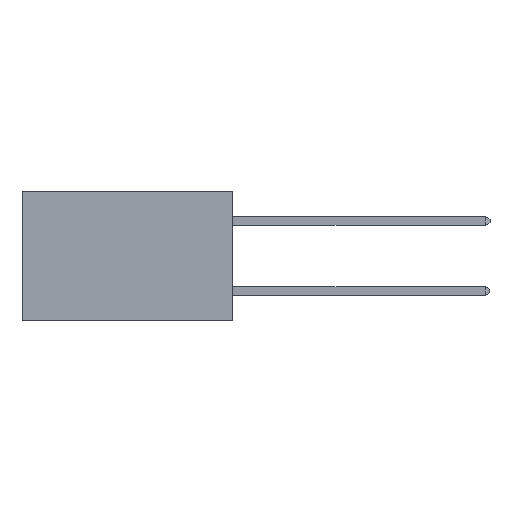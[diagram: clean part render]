
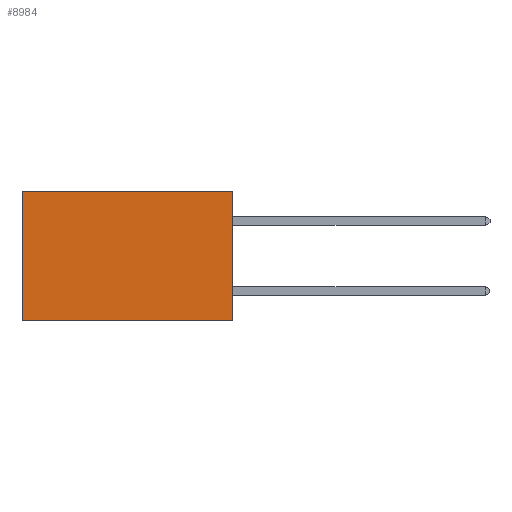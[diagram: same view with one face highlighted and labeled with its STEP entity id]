
A CAD part, left-side view. The second image highlights one B-rep face of the part: STEP entity #8984.
In plain terms, the highlighted planar face has unit normal (-1, 0, 0).
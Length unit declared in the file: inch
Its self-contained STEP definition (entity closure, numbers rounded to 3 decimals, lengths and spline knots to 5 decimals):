
#59 = FACE_OUTER_BOUND ( 'NONE', #17032, .T. ) ;
#88 = VERTEX_POINT ( 'NONE', #13013 ) ;
#177 = LINE ( 'NONE', #3454, #7431 ) ;
#2296 = DIRECTION ( 'NONE',  ( 0., 0., -1. ) ) ;
#2727 = CARTESIAN_POINT ( 'NONE',  ( 0.2875, 0.6, 0. ) ) ;
#3383 = DIRECTION ( 'NONE',  ( 0., 1., 0. ) ) ;
#3454 = CARTESIAN_POINT ( 'NONE',  ( 0.2875, 0., 0. ) ) ;
#4786 = VECTOR ( 'NONE', #8373, 39.37008 ) ;
#5776 = CARTESIAN_POINT ( 'NONE',  ( 0.2875, 0., 0. ) ) ;
#6469 = AXIS2_PLACEMENT_3D ( 'NONE', #5776, #19209, #10375 ) ;
#7085 = VERTEX_POINT ( 'NONE', #18791 ) ;
#7145 = VERTEX_POINT ( 'NONE', #17360 ) ;
#7243 = LINE ( 'NONE', #2727, #11252 ) ;
#7431 = VECTOR ( 'NONE', #3383, 39.37008 ) ;
#8373 = DIRECTION ( 'NONE',  ( 0., 1., 0. ) ) ;
#8984 = ADVANCED_FACE ( 'NONE', ( #59 ), #11770, .F. ) ;
#9493 = ORIENTED_EDGE ( 'NONE', *, *, #11775, .F. ) ;
#10375 = DIRECTION ( 'NONE',  ( 0., 0., -1. ) ) ;
#10382 = DIRECTION ( 'NONE',  ( 0., 0., -1. ) ) ;
#10971 = VECTOR ( 'NONE', #2296, 39.37008 ) ;
#11252 = VECTOR ( 'NONE', #10382, 39.37008 ) ;
#11704 = EDGE_CURVE ( 'NONE', #88, #15437, #12322, .T. ) ;
#11770 = PLANE ( 'NONE',  #6469 ) ;
#11775 = EDGE_CURVE ( 'NONE', #7145, #88, #14912, .T. ) ;
#12322 = LINE ( 'NONE', #17244, #4786 ) ;
#12914 = CARTESIAN_POINT ( 'NONE',  ( 0.2875, 0., 0. ) ) ;
#13013 = CARTESIAN_POINT ( 'NONE',  ( 0.2875, 0., -0.37 ) ) ;
#13158 = EDGE_CURVE ( 'NONE', #7085, #15437, #7243, .T. ) ;
#14912 = LINE ( 'NONE', #12914, #10971 ) ;
#14930 = EDGE_CURVE ( 'NONE', #7145, #7085, #177, .T. ) ;
#15437 = VERTEX_POINT ( 'NONE', #18121 ) ;
#17032 = EDGE_LOOP ( 'NONE', ( #18074, #18758, #9493, #18117 ) ) ;
#17244 = CARTESIAN_POINT ( 'NONE',  ( 0.2875, 0., -0.37 ) ) ;
#17360 = CARTESIAN_POINT ( 'NONE',  ( 0.2875, 0., 0. ) ) ;
#18074 = ORIENTED_EDGE ( 'NONE', *, *, #13158, .T. ) ;
#18117 = ORIENTED_EDGE ( 'NONE', *, *, #14930, .T. ) ;
#18121 = CARTESIAN_POINT ( 'NONE',  ( 0.2875, 0.6, -0.37 ) ) ;
#18758 = ORIENTED_EDGE ( 'NONE', *, *, #11704, .F. ) ;
#18791 = CARTESIAN_POINT ( 'NONE',  ( 0.2875, 0.6, 0. ) ) ;
#19209 = DIRECTION ( 'NONE',  ( 1., 0., 0. ) ) ;
